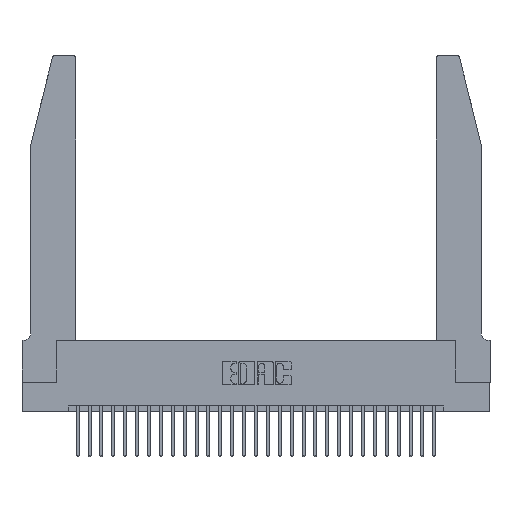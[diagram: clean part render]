
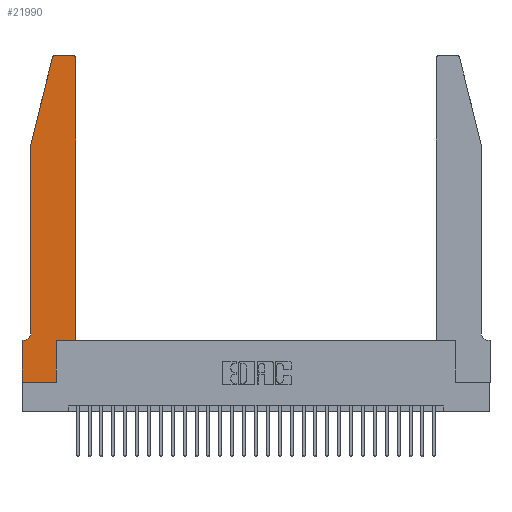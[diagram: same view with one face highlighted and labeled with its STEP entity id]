
A CAD part, top view. The second image highlights one B-rep face of the part: STEP entity #21990.
In plain terms, the highlighted planar face has unit normal (0, 0, 1).
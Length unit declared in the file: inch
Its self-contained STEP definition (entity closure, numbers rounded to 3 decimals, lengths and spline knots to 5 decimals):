
#2 = LINE ( 'NONE', #114, #13402 ) ;
#79 = VECTOR ( 'NONE', #6558, 39.37008 ) ;
#114 = CARTESIAN_POINT ( 'NONE',  ( 0., 0., 0.37 ) ) ;
#374 = CARTESIAN_POINT ( 'NONE',  ( 0.0755, 2., 0.37 ) ) ;
#995 = LINE ( 'NONE', #3828, #19169 ) ;
#2558 = DIRECTION ( 'NONE',  ( 1., 0., 0. ) ) ;
#2653 = CARTESIAN_POINT ( 'NONE',  ( 0.284, 2.75, 0.37 ) ) ;
#3218 = ORIENTED_EDGE ( 'NONE', *, *, #26525, .T. ) ;
#3527 = CARTESIAN_POINT ( 'NONE',  ( 0.4205, 2.75, 0.37 ) ) ;
#3828 = CARTESIAN_POINT ( 'NONE',  ( 0.2605, 2.75, 0.37 ) ) ;
#4185 = DIRECTION ( 'NONE',  ( 0., 0., -1. ) ) ;
#5061 = CARTESIAN_POINT ( 'NONE',  ( 0.0755, 2., 0.37 ) ) ;
#5116 = VERTEX_POINT ( 'NONE', #27509 ) ;
#5190 = VERTEX_POINT ( 'NONE', #27819 ) ;
#5451 = ORIENTED_EDGE ( 'NONE', *, *, #9117, .T. ) ;
#5514 = VECTOR ( 'NONE', #23725, 39.37008 ) ;
#6054 = VERTEX_POINT ( 'NONE', #3527 ) ;
#6284 = PLANE ( 'NONE',  #30251 ) ;
#6367 = CARTESIAN_POINT ( 'NONE',  ( 0.0755, 0.42, 0.37 ) ) ;
#6558 = DIRECTION ( 'NONE',  ( 0., 1., 0. ) ) ;
#6787 = VERTEX_POINT ( 'NONE', #15378 ) ;
#6788 = VERTEX_POINT ( 'NONE', #10721 ) ;
#7001 = VECTOR ( 'NONE', #11043, 39.37008 ) ;
#7143 = ORIENTED_EDGE ( 'NONE', *, *, #11172, .T. ) ;
#7470 = ORIENTED_EDGE ( 'NONE', *, *, #20985, .T. ) ;
#8838 = DIRECTION ( 'NONE',  ( 0., 0., 1. ) ) ;
#8904 = ORIENTED_EDGE ( 'NONE', *, *, #13172, .T. ) ;
#9117 = EDGE_CURVE ( 'NONE', #6788, #5190, #12472, .T. ) ;
#9429 = DIRECTION ( 'NONE',  ( 0., 0., 1. ) ) ;
#9598 = VERTEX_POINT ( 'NONE', #17614 ) ;
#9613 = CARTESIAN_POINT ( 'NONE',  ( 0.4505, 0.35, 0.37 ) ) ;
#9734 = CIRCLE ( 'NONE', #18424, 0.03 ) ;
#10318 = ORIENTED_EDGE ( 'NONE', *, *, #24364, .T. ) ;
#10386 = VECTOR ( 'NONE', #21556, 39.37008 ) ;
#10721 = CARTESIAN_POINT ( 'NONE',  ( 0., 0.35, 0.37 ) ) ;
#11043 = DIRECTION ( 'NONE',  ( 0., -1., 0. ) ) ;
#11124 = LINE ( 'NONE', #5061, #10386 ) ;
#11172 = EDGE_CURVE ( 'NONE', #9598, #21761, #26018, .T. ) ;
#11545 = VECTOR ( 'NONE', #27204, 39.37008 ) ;
#11677 = CARTESIAN_POINT ( 'NONE',  ( 0.2865, 0.35, 0.37 ) ) ;
#12043 = EDGE_CURVE ( 'NONE', #12921, #14190, #21167, .T. ) ;
#12257 = EDGE_CURVE ( 'NONE', #21112, #6787, #9734, .T. ) ;
#12472 = LINE ( 'NONE', #25193, #7001 ) ;
#12921 = VERTEX_POINT ( 'NONE', #18467 ) ;
#13172 = EDGE_CURVE ( 'NONE', #6787, #12921, #11124, .T. ) ;
#13402 = VECTOR ( 'NONE', #2558, 39.37008 ) ;
#14190 = VERTEX_POINT ( 'NONE', #6367 ) ;
#14260 = AXIS2_PLACEMENT_3D ( 'NONE', #18319, #4185, #20690 ) ;
#14888 = VECTOR ( 'NONE', #21717, 39.37008 ) ;
#15378 = CARTESIAN_POINT ( 'NONE',  ( 0.25487, 2.72718, 0.37 ) ) ;
#15592 = DIRECTION ( 'NONE',  ( -1., 0., 0. ) ) ;
#15739 = DIRECTION ( 'NONE',  ( 1., 0., 0. ) ) ;
#17293 = LINE ( 'NONE', #9613, #5514 ) ;
#17614 = CARTESIAN_POINT ( 'NONE',  ( 0.4505, 0.35, 0.37 ) ) ;
#17741 = EDGE_CURVE ( 'NONE', #23996, #25419, #29228, .T. ) ;
#17828 = CARTESIAN_POINT ( 'NONE',  ( 0.0755, 0.35, 0.37 ) ) ;
#18319 = CARTESIAN_POINT ( 'NONE',  ( 0.0055, 0.42, 0.37 ) ) ;
#18424 = AXIS2_PLACEMENT_3D ( 'NONE', #22945, #8838, #25326 ) ;
#18467 = CARTESIAN_POINT ( 'NONE',  ( 0.0755, 2., 0.37 ) ) ;
#19169 = VECTOR ( 'NONE', #15592, 39.37008 ) ;
#20127 = CARTESIAN_POINT ( 'NONE',  ( 0.2865, 0., 0.37 ) ) ;
#20173 = EDGE_CURVE ( 'NONE', #14190, #5116, #23434, .T. ) ;
#20678 = ORIENTED_EDGE ( 'NONE', *, *, #12257, .T. ) ;
#20690 = DIRECTION ( 'NONE',  ( -1., 0., 0. ) ) ;
#20764 = CARTESIAN_POINT ( 'NONE',  ( 0.2865, 0.35, 0.37 ) ) ;
#20901 = ORIENTED_EDGE ( 'NONE', *, *, #17741, .T. ) ;
#20985 = EDGE_CURVE ( 'NONE', #21761, #6054, #26319, .T. ) ;
#21112 = VERTEX_POINT ( 'NONE', #2653 ) ;
#21167 = LINE ( 'NONE', #374, #14888 ) ;
#21556 = DIRECTION ( 'NONE',  ( -0.239, -0.971, 0. ) ) ;
#21717 = DIRECTION ( 'NONE',  ( 0., -1., 0. ) ) ;
#21761 = VERTEX_POINT ( 'NONE', #24310 ) ;
#21990 = ADVANCED_FACE ( 'NONE', ( #30267 ), #6284, .T. ) ;
#22945 = CARTESIAN_POINT ( 'NONE',  ( 0.284, 2.72, 0.37 ) ) ;
#23010 = VECTOR ( 'NONE', #28161, 39.37008 ) ;
#23434 = CIRCLE ( 'NONE', #14260, 0.07 ) ;
#23536 = CARTESIAN_POINT ( 'NONE',  ( 0.4205, 2.72, 0.37 ) ) ;
#23646 = ORIENTED_EDGE ( 'NONE', *, *, #26808, .T. ) ;
#23725 = DIRECTION ( 'NONE',  ( 1., 0., 0. ) ) ;
#23996 = VERTEX_POINT ( 'NONE', #20127 ) ;
#24055 = EDGE_CURVE ( 'NONE', #6054, #21112, #995, .T. ) ;
#24310 = CARTESIAN_POINT ( 'NONE',  ( 0.4505, 2.72, 0.37 ) ) ;
#24364 = EDGE_CURVE ( 'NONE', #25419, #9598, #17293, .T. ) ;
#25193 = CARTESIAN_POINT ( 'NONE',  ( 0., 0., 0.37 ) ) ;
#25326 = DIRECTION ( 'NONE',  ( 1., 0., 0. ) ) ;
#25419 = VERTEX_POINT ( 'NONE', #20764 ) ;
#25492 = ORIENTED_EDGE ( 'NONE', *, *, #24055, .T. ) ;
#25760 = AXIS2_PLACEMENT_3D ( 'NONE', #23536, #9429, #25899 ) ;
#25899 = DIRECTION ( 'NONE',  ( 1., 0., 0. ) ) ;
#26018 = LINE ( 'NONE', #27853, #79 ) ;
#26319 = CIRCLE ( 'NONE', #25760, 0.03 ) ;
#26525 = EDGE_CURVE ( 'NONE', #5190, #23996, #2, .T. ) ;
#26808 = EDGE_CURVE ( 'NONE', #5116, #6788, #29569, .T. ) ;
#27204 = DIRECTION ( 'NONE',  ( -1., 0., 0. ) ) ;
#27478 = CARTESIAN_POINT ( 'NONE',  ( 0., 0.35, 0.37 ) ) ;
#27509 = CARTESIAN_POINT ( 'NONE',  ( 0.0055, 0.35, 0.37 ) ) ;
#27693 = ORIENTED_EDGE ( 'NONE', *, *, #12043, .T. ) ;
#27819 = CARTESIAN_POINT ( 'NONE',  ( 0., 0., 0.37 ) ) ;
#27853 = CARTESIAN_POINT ( 'NONE',  ( 0.4505, 0.35, 0.37 ) ) ;
#28161 = DIRECTION ( 'NONE',  ( 0., 1., 0. ) ) ;
#28411 = ORIENTED_EDGE ( 'NONE', *, *, #20173, .T. ) ;
#29228 = LINE ( 'NONE', #11677, #23010 ) ;
#29569 = LINE ( 'NONE', #17828, #11545 ) ;
#29804 = DIRECTION ( 'NONE',  ( 0., 0., 1. ) ) ;
#29807 = EDGE_LOOP ( 'NONE', ( #25492, #20678, #8904, #27693, #28411, #23646, #5451, #3218, #20901, #10318, #7143, #7470 ) ) ;
#30251 = AXIS2_PLACEMENT_3D ( 'NONE', #27478, #29804, #15739 ) ;
#30267 = FACE_OUTER_BOUND ( 'NONE', #29807, .T. ) ;
